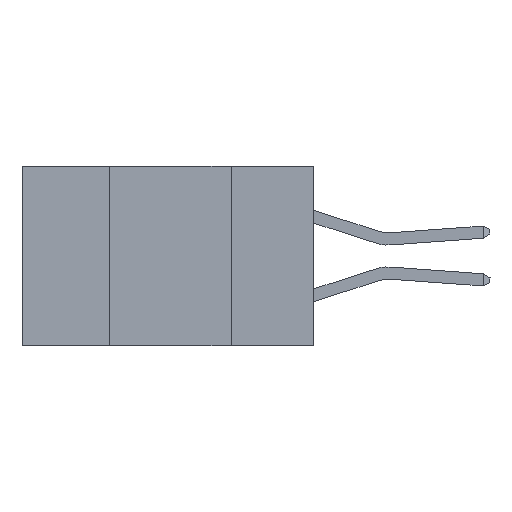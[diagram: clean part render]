
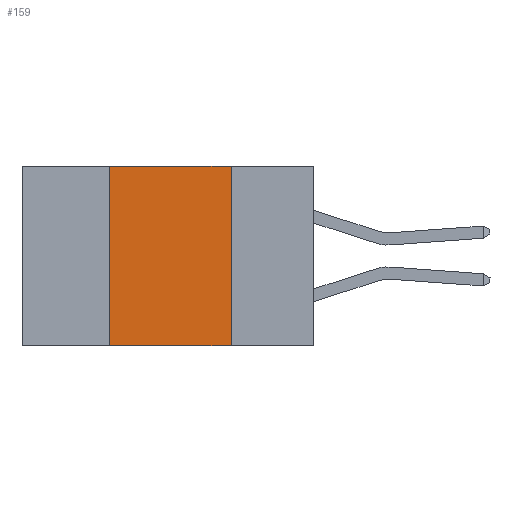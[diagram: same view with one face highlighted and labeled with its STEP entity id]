
A CAD part, left-side view. The second image highlights one B-rep face of the part: STEP entity #159.
In plain terms, the highlighted planar face has unit normal (-1, 0, 0).
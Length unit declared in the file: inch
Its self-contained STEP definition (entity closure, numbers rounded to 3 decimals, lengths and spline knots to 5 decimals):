
#159 = ADVANCED_FACE ( 'NONE', ( #2785 ), #7889, .F. ) ;
#1942 = CARTESIAN_POINT ( 'NONE',  ( 0., 0.42, -0.37 ) ) ;
#2298 = LINE ( 'NONE', #10381, #3420 ) ;
#2785 = FACE_OUTER_BOUND ( 'NONE', #6335, .T. ) ;
#3357 = LINE ( 'NONE', #5079, #8400 ) ;
#3420 = VECTOR ( 'NONE', #17876, 39.37008 ) ;
#4513 = VERTEX_POINT ( 'NONE', #1942 ) ;
#5079 = CARTESIAN_POINT ( 'NONE',  ( 0., 0.6, 0. ) ) ;
#5478 = CARTESIAN_POINT ( 'NONE',  ( 0., 0.42, 0. ) ) ;
#5840 = VERTEX_POINT ( 'NONE', #8365 ) ;
#6335 = EDGE_LOOP ( 'NONE', ( #20798, #20228, #23107, #19593 ) ) ;
#6350 = AXIS2_PLACEMENT_3D ( 'NONE', #9714, #20369, #9553 ) ;
#6421 = EDGE_CURVE ( 'NONE', #4513, #7576, #7892, .T. ) ;
#7495 = DIRECTION ( 'NONE',  ( 0., -1., 0. ) ) ;
#7576 = VERTEX_POINT ( 'NONE', #19213 ) ;
#7889 = PLANE ( 'NONE',  #6350 ) ;
#7892 = LINE ( 'NONE', #9121, #22327 ) ;
#8290 = VERTEX_POINT ( 'NONE', #5478 ) ;
#8365 = CARTESIAN_POINT ( 'NONE',  ( 0., 0.17, 0. ) ) ;
#8400 = VECTOR ( 'NONE', #7495, 39.37008 ) ;
#9121 = CARTESIAN_POINT ( 'NONE',  ( 0., 0.6, -0.37 ) ) ;
#9553 = DIRECTION ( 'NONE',  ( 0., 0., -1. ) ) ;
#9714 = CARTESIAN_POINT ( 'NONE',  ( 0., 0.6, 0. ) ) ;
#10381 = CARTESIAN_POINT ( 'NONE',  ( 0., 0.17, 0. ) ) ;
#12590 = EDGE_CURVE ( 'NONE', #8290, #5840, #3357, .T. ) ;
#12999 = DIRECTION ( 'NONE',  ( 0., 0., 1. ) ) ;
#14259 = DIRECTION ( 'NONE',  ( 0., -1., 0. ) ) ;
#15866 = VECTOR ( 'NONE', #12999, 39.37008 ) ;
#16073 = EDGE_CURVE ( 'NONE', #4513, #8290, #20922, .T. ) ;
#17876 = DIRECTION ( 'NONE',  ( 0., 0., -1. ) ) ;
#18419 = CARTESIAN_POINT ( 'NONE',  ( 0., 0.42, 0. ) ) ;
#19213 = CARTESIAN_POINT ( 'NONE',  ( 0., 0.17, -0.37 ) ) ;
#19593 = ORIENTED_EDGE ( 'NONE', *, *, #6421, .T. ) ;
#20228 = ORIENTED_EDGE ( 'NONE', *, *, #12590, .F. ) ;
#20369 = DIRECTION ( 'NONE',  ( 1., 0., 0. ) ) ;
#20655 = EDGE_CURVE ( 'NONE', #5840, #7576, #2298, .T. ) ;
#20798 = ORIENTED_EDGE ( 'NONE', *, *, #20655, .F. ) ;
#20922 = LINE ( 'NONE', #18419, #15866 ) ;
#22327 = VECTOR ( 'NONE', #14259, 39.37008 ) ;
#23107 = ORIENTED_EDGE ( 'NONE', *, *, #16073, .F. ) ;
